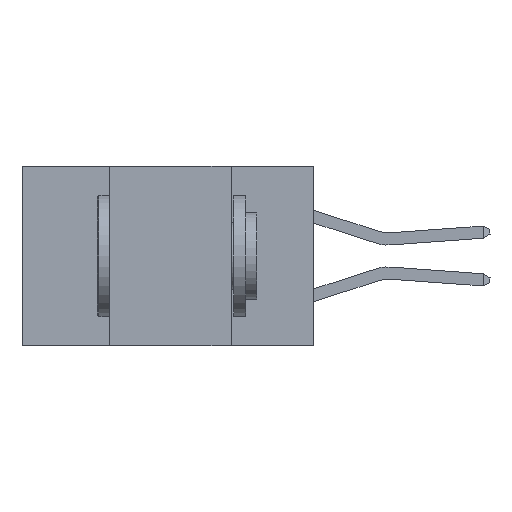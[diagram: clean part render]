
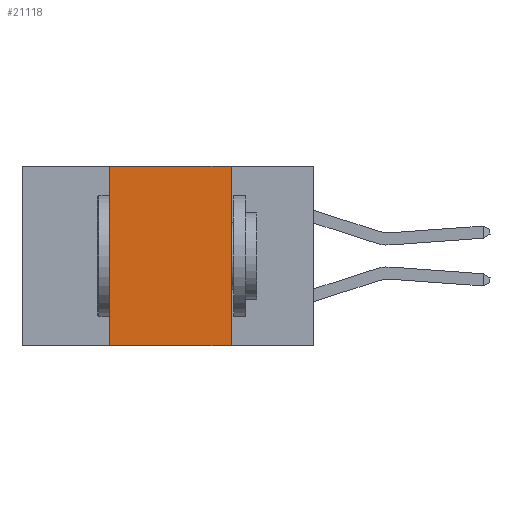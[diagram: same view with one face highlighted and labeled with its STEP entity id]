
A CAD part, left-side view. The second image highlights one B-rep face of the part: STEP entity #21118.
In plain terms, the highlighted planar face has unit normal (-1, 0, 0).
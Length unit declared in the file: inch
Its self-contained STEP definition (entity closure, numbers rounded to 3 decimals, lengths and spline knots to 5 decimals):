
#449 = LINE ( 'NONE', #9573, #20250 ) ;
#455 = DIRECTION ( 'NONE',  ( 1., 0., 0. ) ) ;
#1612 = VECTOR ( 'NONE', #4193, 39.37008 ) ;
#2027 = VECTOR ( 'NONE', #4417, 39.37008 ) ;
#2503 = CARTESIAN_POINT ( 'NONE',  ( 0., 0.17, 0. ) ) ;
#3738 = EDGE_LOOP ( 'NONE', ( #18934, #17113, #21827, #5722 ) ) ;
#4193 = DIRECTION ( 'NONE',  ( 0., -1., 0. ) ) ;
#4413 = DIRECTION ( 'NONE',  ( 0., 0., -1. ) ) ;
#4417 = DIRECTION ( 'NONE',  ( 0., 0., -1. ) ) ;
#4763 = VECTOR ( 'NONE', #19527, 39.37008 ) ;
#5722 = ORIENTED_EDGE ( 'NONE', *, *, #8643, .T. ) ;
#6335 = EDGE_CURVE ( 'NONE', #21741, #13705, #22116, .T. ) ;
#6570 = CARTESIAN_POINT ( 'NONE',  ( 0., 0.17, 0. ) ) ;
#6759 = CARTESIAN_POINT ( 'NONE',  ( 0., 0.17, -0.37 ) ) ;
#8643 = EDGE_CURVE ( 'NONE', #20863, #13705, #15252, .T. ) ;
#8678 = AXIS2_PLACEMENT_3D ( 'NONE', #9799, #455, #4413 ) ;
#8933 = EDGE_CURVE ( 'NONE', #20863, #11503, #18724, .T. ) ;
#9573 = CARTESIAN_POINT ( 'NONE',  ( 0., 0.6, 0. ) ) ;
#9799 = CARTESIAN_POINT ( 'NONE',  ( 0., 0.6, 0. ) ) ;
#11503 = VERTEX_POINT ( 'NONE', #21614 ) ;
#12974 = FACE_OUTER_BOUND ( 'NONE', #3738, .T. ) ;
#13642 = CARTESIAN_POINT ( 'NONE',  ( 0., 0.6, -0.37 ) ) ;
#13705 = VERTEX_POINT ( 'NONE', #6759 ) ;
#15252 = LINE ( 'NONE', #13642, #1612 ) ;
#15783 = CARTESIAN_POINT ( 'NONE',  ( 0., 0.42, 0. ) ) ;
#16937 = CARTESIAN_POINT ( 'NONE',  ( 0., 0.42, -0.37 ) ) ;
#17113 = ORIENTED_EDGE ( 'NONE', *, *, #21690, .F. ) ;
#18724 = LINE ( 'NONE', #15783, #4763 ) ;
#18934 = ORIENTED_EDGE ( 'NONE', *, *, #6335, .F. ) ;
#19063 = PLANE ( 'NONE',  #8678 ) ;
#19527 = DIRECTION ( 'NONE',  ( 0., 0., 1. ) ) ;
#20250 = VECTOR ( 'NONE', #22391, 39.37008 ) ;
#20863 = VERTEX_POINT ( 'NONE', #16937 ) ;
#21118 = ADVANCED_FACE ( 'NONE', ( #12974 ), #19063, .F. ) ;
#21614 = CARTESIAN_POINT ( 'NONE',  ( 0., 0.42, 0. ) ) ;
#21690 = EDGE_CURVE ( 'NONE', #11503, #21741, #449, .T. ) ;
#21741 = VERTEX_POINT ( 'NONE', #2503 ) ;
#21827 = ORIENTED_EDGE ( 'NONE', *, *, #8933, .F. ) ;
#22116 = LINE ( 'NONE', #6570, #2027 ) ;
#22391 = DIRECTION ( 'NONE',  ( 0., -1., 0. ) ) ;
